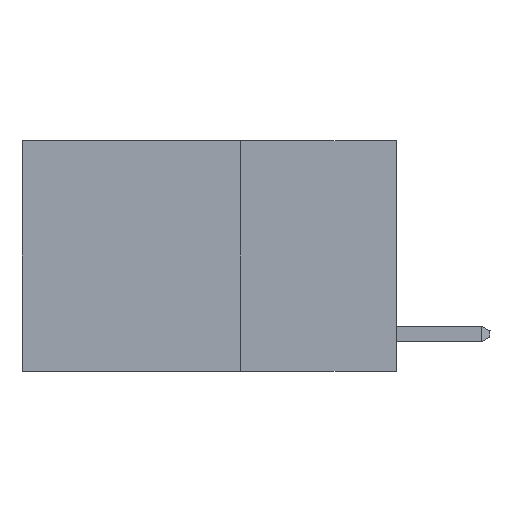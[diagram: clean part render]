
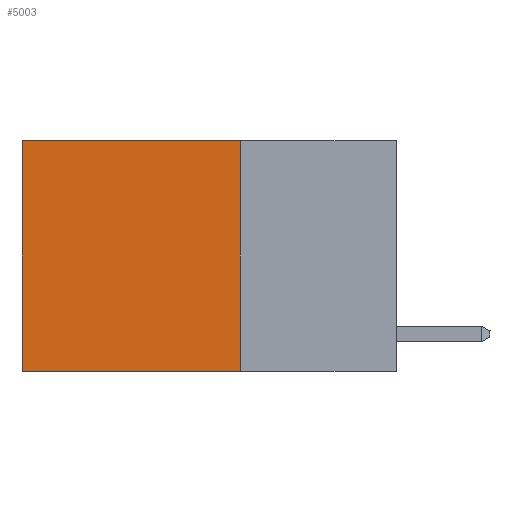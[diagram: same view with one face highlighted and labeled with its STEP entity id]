
A CAD part, left-side view. The second image highlights one B-rep face of the part: STEP entity #5003.
In plain terms, the highlighted planar face has unit normal (-1, 0, 0).
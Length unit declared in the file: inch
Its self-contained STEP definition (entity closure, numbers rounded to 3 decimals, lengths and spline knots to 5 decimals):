
#76 = ORIENTED_EDGE ( 'NONE', *, *, #4659, .T. ) ;
#551 = PLANE ( 'NONE',  #4033 ) ;
#710 = ORIENTED_EDGE ( 'NONE', *, *, #7168, .F. ) ;
#902 = LINE ( 'NONE', #5361, #9253 ) ;
#2114 = DIRECTION ( 'NONE',  ( 0., 1., 0. ) ) ;
#2117 = ORIENTED_EDGE ( 'NONE', *, *, #8183, .T. ) ;
#2433 = LINE ( 'NONE', #7226, #3633 ) ;
#2709 = VERTEX_POINT ( 'NONE', #11424 ) ;
#2821 = DIRECTION ( 'NONE',  ( 1., 0., 0. ) ) ;
#3000 = CARTESIAN_POINT ( 'NONE',  ( 0.2625, 0.25, 0. ) ) ;
#3325 = VECTOR ( 'NONE', #3780, 39.37008 ) ;
#3479 = EDGE_LOOP ( 'NONE', ( #2117, #9934, #710, #76 ) ) ;
#3633 = VECTOR ( 'NONE', #12441, 39.37008 ) ;
#3780 = DIRECTION ( 'NONE',  ( 0., 0., -1. ) ) ;
#4033 = AXIS2_PLACEMENT_3D ( 'NONE', #12848, #2821, #7273 ) ;
#4065 = LINE ( 'NONE', #10735, #5518 ) ;
#4480 = EDGE_CURVE ( 'NONE', #2709, #11449, #2433, .T. ) ;
#4659 = EDGE_CURVE ( 'NONE', #6030, #6459, #4065, .T. ) ;
#4730 = LINE ( 'NONE', #9188, #3325 ) ;
#5003 = ADVANCED_FACE ( 'NONE', ( #8230 ), #551, .F. ) ;
#5361 = CARTESIAN_POINT ( 'NONE',  ( 0.2625, 0.25, 0. ) ) ;
#5518 = VECTOR ( 'NONE', #2114, 39.37008 ) ;
#6030 = VERTEX_POINT ( 'NONE', #3000 ) ;
#6459 = VERTEX_POINT ( 'NONE', #9711 ) ;
#6679 = DIRECTION ( 'NONE',  ( 0., 0., -1. ) ) ;
#7168 = EDGE_CURVE ( 'NONE', #6030, #2709, #902, .T. ) ;
#7226 = CARTESIAN_POINT ( 'NONE',  ( 0.2625, 0.25, -0.37 ) ) ;
#7273 = DIRECTION ( 'NONE',  ( 0., 0., -1. ) ) ;
#8183 = EDGE_CURVE ( 'NONE', #6459, #11449, #4730, .T. ) ;
#8230 = FACE_OUTER_BOUND ( 'NONE', #3479, .T. ) ;
#9188 = CARTESIAN_POINT ( 'NONE',  ( 0.2625, 0.6, 0. ) ) ;
#9253 = VECTOR ( 'NONE', #6679, 39.37008 ) ;
#9711 = CARTESIAN_POINT ( 'NONE',  ( 0.2625, 0.6, 0. ) ) ;
#9934 = ORIENTED_EDGE ( 'NONE', *, *, #4480, .F. ) ;
#10017 = CARTESIAN_POINT ( 'NONE',  ( 0.2625, 0.6, -0.37 ) ) ;
#10735 = CARTESIAN_POINT ( 'NONE',  ( 0.2625, 0.25, 0. ) ) ;
#11424 = CARTESIAN_POINT ( 'NONE',  ( 0.2625, 0.25, -0.37 ) ) ;
#11449 = VERTEX_POINT ( 'NONE', #10017 ) ;
#12441 = DIRECTION ( 'NONE',  ( 0., 1., 0. ) ) ;
#12848 = CARTESIAN_POINT ( 'NONE',  ( 0.2625, 0.25, 0. ) ) ;
